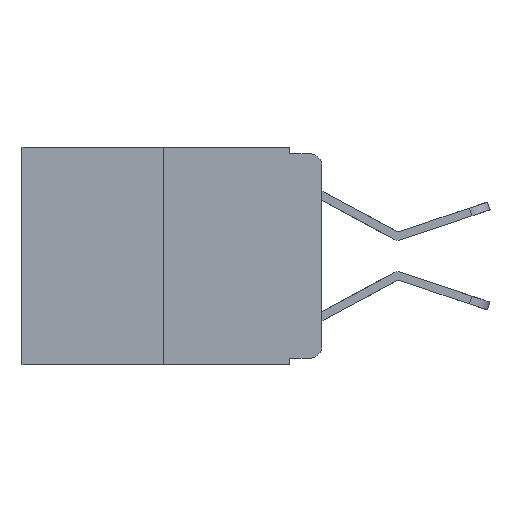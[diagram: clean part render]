
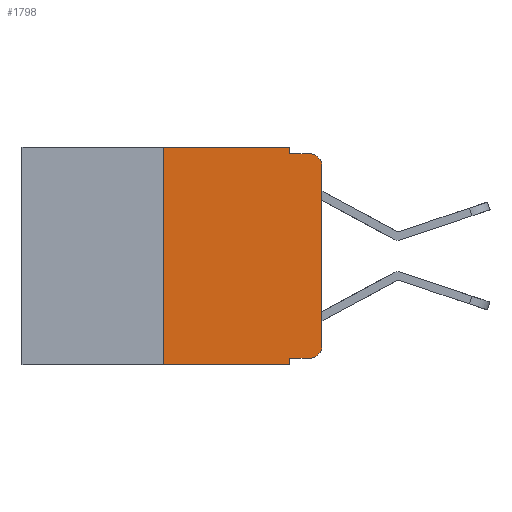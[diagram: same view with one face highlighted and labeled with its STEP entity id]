
A CAD part, left-side view. The second image highlights one B-rep face of the part: STEP entity #1798.
In plain terms, the highlighted planar face has unit normal (-1, 0, 0).
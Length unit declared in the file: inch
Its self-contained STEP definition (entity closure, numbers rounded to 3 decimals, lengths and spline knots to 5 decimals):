
#179 = VERTEX_POINT ( 'NONE', #4146 ) ;
#234 = VECTOR ( 'NONE', #10893, 39.37008 ) ;
#542 = LINE ( 'NONE', #11022, #234 ) ;
#609 = DIRECTION ( 'NONE',  ( 0., 0., -1. ) ) ;
#661 = VERTEX_POINT ( 'NONE', #2807 ) ;
#713 = CIRCLE ( 'NONE', #4766, 0.02 ) ;
#1333 = VERTEX_POINT ( 'NONE', #9336 ) ;
#1643 = ORIENTED_EDGE ( 'NONE', *, *, #6454, .F. ) ;
#1748 = VECTOR ( 'NONE', #2183, 39.37008 ) ;
#1798 = ADVANCED_FACE ( 'NONE', ( #4414 ), #11025, .F. ) ;
#2183 = DIRECTION ( 'NONE',  ( 0., -1., 0. ) ) ;
#2381 = EDGE_LOOP ( 'NONE', ( #9718, #5771, #8421, #7156, #1643, #2579, #11280, #6178, #9866, #4669 ) ) ;
#2579 = ORIENTED_EDGE ( 'NONE', *, *, #4334, .F. ) ;
#2807 = CARTESIAN_POINT ( 'NONE',  ( 0., 0.051, 0. ) ) ;
#2971 = EDGE_CURVE ( 'NONE', #5586, #3982, #5118, .T. ) ;
#3144 = CARTESIAN_POINT ( 'NONE',  ( 0., 0.473, 0. ) ) ;
#3307 = CARTESIAN_POINT ( 'NONE',  ( 0., 0.02, -0.01 ) ) ;
#3330 = VECTOR ( 'NONE', #10100, 39.37008 ) ;
#3475 = VECTOR ( 'NONE', #11149, 39.37008 ) ;
#3649 = VERTEX_POINT ( 'NONE', #6811 ) ;
#3760 = VERTEX_POINT ( 'NONE', #3307 ) ;
#3982 = VERTEX_POINT ( 'NONE', #10470 ) ;
#4106 = EDGE_CURVE ( 'NONE', #4894, #3760, #8133, .T. ) ;
#4110 = EDGE_CURVE ( 'NONE', #1333, #4894, #8662, .T. ) ;
#4125 = EDGE_CURVE ( 'NONE', #179, #1333, #713, .T. ) ;
#4146 = CARTESIAN_POINT ( 'NONE',  ( 0., 0.02, -0.333 ) ) ;
#4189 = EDGE_CURVE ( 'NONE', #661, #4847, #7288, .T. ) ;
#4211 = EDGE_CURVE ( 'NONE', #4847, #3760, #11264, .T. ) ;
#4224 = DIRECTION ( 'NONE',  ( -1., 0., 0. ) ) ;
#4317 = EDGE_CURVE ( 'NONE', #4438, #179, #10241, .T. ) ;
#4319 = EDGE_CURVE ( 'NONE', #4438, #3982, #6436, .T. ) ;
#4334 = EDGE_CURVE ( 'NONE', #5586, #3649, #542, .T. ) ;
#4414 = FACE_OUTER_BOUND ( 'NONE', #2381, .T. ) ;
#4438 = VERTEX_POINT ( 'NONE', #9460 ) ;
#4470 = DIRECTION ( 'NONE',  ( 0., -1., 0. ) ) ;
#4669 = ORIENTED_EDGE ( 'NONE', *, *, #4125, .T. ) ;
#4766 = AXIS2_PLACEMENT_3D ( 'NONE', #5915, #4224, #609 ) ;
#4847 = VERTEX_POINT ( 'NONE', #10562 ) ;
#4894 = VERTEX_POINT ( 'NONE', #6478 ) ;
#4972 = AXIS2_PLACEMENT_3D ( 'NONE', #10917, #10956, #10468 ) ;
#5074 = CARTESIAN_POINT ( 'NONE',  ( 0., 0.051, -0.333 ) ) ;
#5118 = LINE ( 'NONE', #5147, #11683 ) ;
#5147 = CARTESIAN_POINT ( 'NONE',  ( 0., 0.473, -0.343 ) ) ;
#5586 = VERTEX_POINT ( 'NONE', #5674 ) ;
#5674 = CARTESIAN_POINT ( 'NONE',  ( 0., 0.25, -0.343 ) ) ;
#5771 = ORIENTED_EDGE ( 'NONE', *, *, #4106, .T. ) ;
#5915 = CARTESIAN_POINT ( 'NONE',  ( 0., 0.02, -0.313 ) ) ;
#5945 = AXIS2_PLACEMENT_3D ( 'NONE', #9430, #6770, #8443 ) ;
#6178 = ORIENTED_EDGE ( 'NONE', *, *, #4319, .F. ) ;
#6436 = LINE ( 'NONE', #8018, #3475 ) ;
#6454 = EDGE_CURVE ( 'NONE', #3649, #661, #11236, .T. ) ;
#6478 = CARTESIAN_POINT ( 'NONE',  ( 0., 0., -0.03 ) ) ;
#6521 = CARTESIAN_POINT ( 'NONE',  ( 0., 0., 0. ) ) ;
#6770 = DIRECTION ( 'NONE',  ( -1., 0., 0. ) ) ;
#6811 = CARTESIAN_POINT ( 'NONE',  ( 0., 0.25, 0. ) ) ;
#7018 = VECTOR ( 'NONE', #8387, 39.37008 ) ;
#7156 = ORIENTED_EDGE ( 'NONE', *, *, #4189, .F. ) ;
#7288 = LINE ( 'NONE', #8878, #7018 ) ;
#7745 = DIRECTION ( 'NONE',  ( 0., -1., 0. ) ) ;
#7992 = VECTOR ( 'NONE', #11468, 39.37008 ) ;
#8018 = CARTESIAN_POINT ( 'NONE',  ( 0., 0.051, 0. ) ) ;
#8133 = CIRCLE ( 'NONE', #5945, 0.02 ) ;
#8387 = DIRECTION ( 'NONE',  ( 0., 0., -1. ) ) ;
#8421 = ORIENTED_EDGE ( 'NONE', *, *, #4211, .F. ) ;
#8443 = DIRECTION ( 'NONE',  ( 0., 0., -1. ) ) ;
#8662 = LINE ( 'NONE', #6521, #3330 ) ;
#8794 = CARTESIAN_POINT ( 'NONE',  ( 0., 0.051, -0.01 ) ) ;
#8878 = CARTESIAN_POINT ( 'NONE',  ( 0., 0.051, 0. ) ) ;
#9336 = CARTESIAN_POINT ( 'NONE',  ( 0., 0., -0.313 ) ) ;
#9430 = CARTESIAN_POINT ( 'NONE',  ( 0., 0.02, -0.03 ) ) ;
#9460 = CARTESIAN_POINT ( 'NONE',  ( 0., 0.051, -0.333 ) ) ;
#9718 = ORIENTED_EDGE ( 'NONE', *, *, #4110, .T. ) ;
#9866 = ORIENTED_EDGE ( 'NONE', *, *, #4317, .T. ) ;
#10100 = DIRECTION ( 'NONE',  ( 0., 0., 1. ) ) ;
#10241 = LINE ( 'NONE', #5074, #7992 ) ;
#10468 = DIRECTION ( 'NONE',  ( 0., 0., -1. ) ) ;
#10470 = CARTESIAN_POINT ( 'NONE',  ( 0., 0.051, -0.343 ) ) ;
#10562 = CARTESIAN_POINT ( 'NONE',  ( 0., 0.051, -0.01 ) ) ;
#10893 = DIRECTION ( 'NONE',  ( 0., 0., 1. ) ) ;
#10917 = CARTESIAN_POINT ( 'NONE',  ( 0., 0.473, 0. ) ) ;
#10956 = DIRECTION ( 'NONE',  ( 1., 0., 0. ) ) ;
#11009 = VECTOR ( 'NONE', #7745, 39.37008 ) ;
#11022 = CARTESIAN_POINT ( 'NONE',  ( 0., 0.25, 0. ) ) ;
#11025 = PLANE ( 'NONE',  #4972 ) ;
#11149 = DIRECTION ( 'NONE',  ( 0., 0., -1. ) ) ;
#11236 = LINE ( 'NONE', #3144, #1748 ) ;
#11264 = LINE ( 'NONE', #8794, #11009 ) ;
#11280 = ORIENTED_EDGE ( 'NONE', *, *, #2971, .T. ) ;
#11468 = DIRECTION ( 'NONE',  ( 0., -1., 0. ) ) ;
#11683 = VECTOR ( 'NONE', #4470, 39.37008 ) ;
